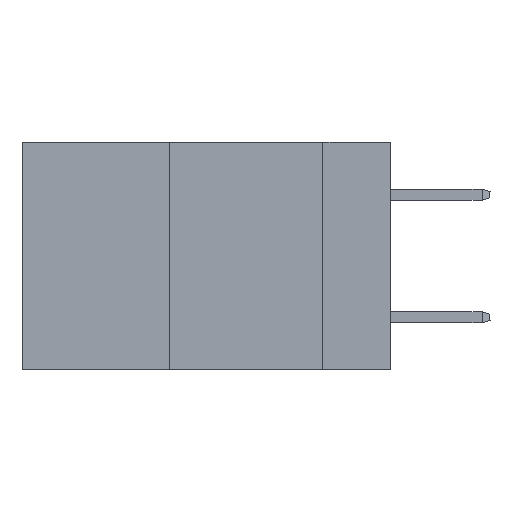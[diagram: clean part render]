
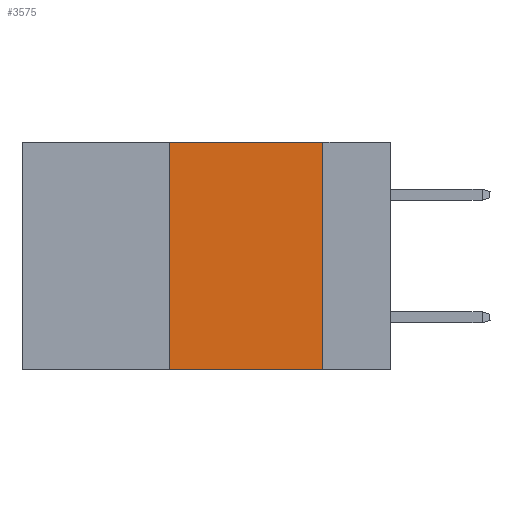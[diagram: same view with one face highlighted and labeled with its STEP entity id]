
A CAD part, left-side view. The second image highlights one B-rep face of the part: STEP entity #3575.
In plain terms, the highlighted planar face has unit normal (-1, 0, 0).
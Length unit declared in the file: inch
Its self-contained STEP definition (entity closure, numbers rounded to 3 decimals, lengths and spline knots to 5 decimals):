
#729 = VERTEX_POINT ( 'NONE', #10705 ) ;
#2086 = DIRECTION ( 'NONE',  ( 0., 0., -1. ) ) ;
#2468 = CARTESIAN_POINT ( 'NONE',  ( 0., 0.36, -0.37 ) ) ;
#3575 = ADVANCED_FACE ( 'NONE', ( #18408 ), #16830, .F. ) ;
#5446 = VERTEX_POINT ( 'NONE', #18351 ) ;
#5724 = CARTESIAN_POINT ( 'NONE',  ( 0., 0.6, 0. ) ) ;
#5738 = CARTESIAN_POINT ( 'NONE',  ( 0., 0.36, 0. ) ) ;
#7578 = DIRECTION ( 'NONE',  ( 1., 0., 0. ) ) ;
#9008 = EDGE_CURVE ( 'NONE', #20249, #5446, #14567, .T. ) ;
#9641 = VECTOR ( 'NONE', #16926, 39.37008 ) ;
#9961 = LINE ( 'NONE', #13838, #20682 ) ;
#10001 = ORIENTED_EDGE ( 'NONE', *, *, #20253, .F. ) ;
#10705 = CARTESIAN_POINT ( 'NONE',  ( 0., 0.11, -0.37 ) ) ;
#11950 = CARTESIAN_POINT ( 'NONE',  ( 0., 0.11, 0. ) ) ;
#12822 = ORIENTED_EDGE ( 'NONE', *, *, #19672, .T. ) ;
#13582 = CARTESIAN_POINT ( 'NONE',  ( 0., 0.6, 0. ) ) ;
#13702 = VECTOR ( 'NONE', #21371, 39.37008 ) ;
#13838 = CARTESIAN_POINT ( 'NONE',  ( 0., 0.6, -0.37 ) ) ;
#14567 = LINE ( 'NONE', #5738, #9641 ) ;
#16830 = PLANE ( 'NONE',  #21877 ) ;
#16885 = DIRECTION ( 'NONE',  ( 0., -1., 0. ) ) ;
#16926 = DIRECTION ( 'NONE',  ( 0., 0., 1. ) ) ;
#17418 = LINE ( 'NONE', #13582, #20576 ) ;
#17768 = EDGE_LOOP ( 'NONE', ( #18671, #10001, #18209, #12822 ) ) ;
#18196 = VERTEX_POINT ( 'NONE', #20494 ) ;
#18209 = ORIENTED_EDGE ( 'NONE', *, *, #9008, .F. ) ;
#18351 = CARTESIAN_POINT ( 'NONE',  ( 0., 0.36, 0. ) ) ;
#18408 = FACE_OUTER_BOUND ( 'NONE', #17768, .T. ) ;
#18435 = EDGE_CURVE ( 'NONE', #18196, #729, #19162, .T. ) ;
#18671 = ORIENTED_EDGE ( 'NONE', *, *, #18435, .F. ) ;
#19162 = LINE ( 'NONE', #11950, #13702 ) ;
#19672 = EDGE_CURVE ( 'NONE', #20249, #729, #9961, .T. ) ;
#20249 = VERTEX_POINT ( 'NONE', #2468 ) ;
#20253 = EDGE_CURVE ( 'NONE', #5446, #18196, #17418, .T. ) ;
#20494 = CARTESIAN_POINT ( 'NONE',  ( 0., 0.11, 0. ) ) ;
#20576 = VECTOR ( 'NONE', #16885, 39.37008 ) ;
#20682 = VECTOR ( 'NONE', #22782, 39.37008 ) ;
#21371 = DIRECTION ( 'NONE',  ( 0., 0., -1. ) ) ;
#21877 = AXIS2_PLACEMENT_3D ( 'NONE', #5724, #7578, #2086 ) ;
#22782 = DIRECTION ( 'NONE',  ( 0., -1., 0. ) ) ;
